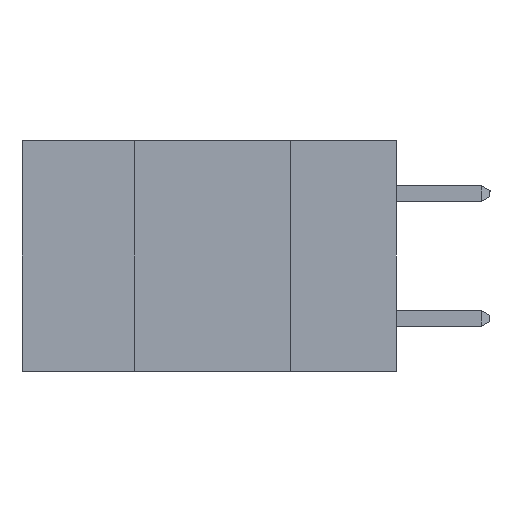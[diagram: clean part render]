
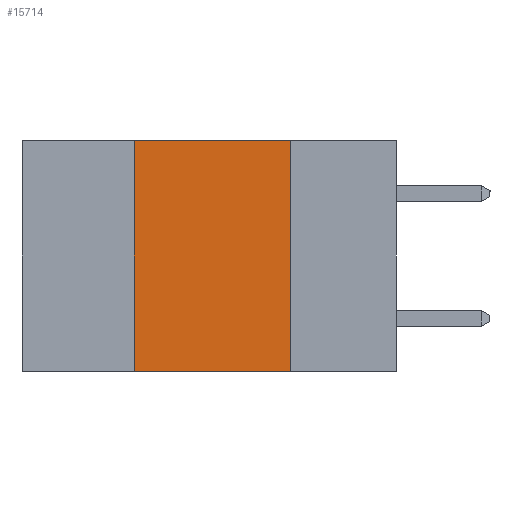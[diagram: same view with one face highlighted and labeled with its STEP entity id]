
A CAD part, left-side view. The second image highlights one B-rep face of the part: STEP entity #15714.
In plain terms, the highlighted planar face has unit normal (-1, 0, 0).
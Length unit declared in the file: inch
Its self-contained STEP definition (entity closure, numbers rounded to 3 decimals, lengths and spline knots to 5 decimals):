
#334 = DIRECTION ( 'NONE',  ( 0., 0., -1. ) ) ;
#841 = LINE ( 'NONE', #19370, #11485 ) ;
#1142 = CARTESIAN_POINT ( 'NONE',  ( 0., 0.17, -0.37 ) ) ;
#1306 = CARTESIAN_POINT ( 'NONE',  ( 0., 0.42, -0.37 ) ) ;
#1556 = DIRECTION ( 'NONE',  ( 0., 0., 1. ) ) ;
#3367 = DIRECTION ( 'NONE',  ( 0., -1., 0. ) ) ;
#3620 = LINE ( 'NONE', #7492, #9750 ) ;
#4658 = CARTESIAN_POINT ( 'NONE',  ( 0., 0.17, 0. ) ) ;
#4849 = DIRECTION ( 'NONE',  ( 0., -1., 0. ) ) ;
#5846 = AXIS2_PLACEMENT_3D ( 'NONE', #8192, #14213, #334 ) ;
#6128 = VERTEX_POINT ( 'NONE', #1142 ) ;
#6526 = ORIENTED_EDGE ( 'NONE', *, *, #19550, .F. ) ;
#7252 = EDGE_CURVE ( 'NONE', #15721, #6128, #3620, .T. ) ;
#7492 = CARTESIAN_POINT ( 'NONE',  ( 0., 0.6, -0.37 ) ) ;
#8192 = CARTESIAN_POINT ( 'NONE',  ( 0., 0.6, 0. ) ) ;
#8269 = EDGE_CURVE ( 'NONE', #10530, #13784, #841, .T. ) ;
#8507 = DIRECTION ( 'NONE',  ( 0., 0., -1. ) ) ;
#9715 = ORIENTED_EDGE ( 'NONE', *, *, #13965, .F. ) ;
#9750 = VECTOR ( 'NONE', #3367, 39.37008 ) ;
#10458 = PLANE ( 'NONE',  #5846 ) ;
#10530 = VERTEX_POINT ( 'NONE', #16294 ) ;
#11485 = VECTOR ( 'NONE', #4849, 39.37008 ) ;
#11869 = VECTOR ( 'NONE', #8507, 39.37008 ) ;
#12522 = LINE ( 'NONE', #16385, #11869 ) ;
#13784 = VERTEX_POINT ( 'NONE', #4658 ) ;
#13965 = EDGE_CURVE ( 'NONE', #15721, #10530, #17711, .T. ) ;
#14213 = DIRECTION ( 'NONE',  ( 1., 0., 0. ) ) ;
#15415 = VECTOR ( 'NONE', #1556, 39.37008 ) ;
#15714 = ADVANCED_FACE ( 'NONE', ( #22861 ), #10458, .F. ) ;
#15721 = VERTEX_POINT ( 'NONE', #16209 ) ;
#16209 = CARTESIAN_POINT ( 'NONE',  ( 0., 0.42, -0.37 ) ) ;
#16294 = CARTESIAN_POINT ( 'NONE',  ( 0., 0.42, 0. ) ) ;
#16385 = CARTESIAN_POINT ( 'NONE',  ( 0., 0.17, -0.37 ) ) ;
#17711 = LINE ( 'NONE', #1306, #15415 ) ;
#19370 = CARTESIAN_POINT ( 'NONE',  ( 0., 0.6, 0. ) ) ;
#19550 = EDGE_CURVE ( 'NONE', #13784, #6128, #12522, .T. ) ;
#20189 = ORIENTED_EDGE ( 'NONE', *, *, #7252, .T. ) ;
#22861 = FACE_OUTER_BOUND ( 'NONE', #25699, .T. ) ;
#25699 = EDGE_LOOP ( 'NONE', ( #6526, #26317, #9715, #20189 ) ) ;
#26317 = ORIENTED_EDGE ( 'NONE', *, *, #8269, .F. ) ;
